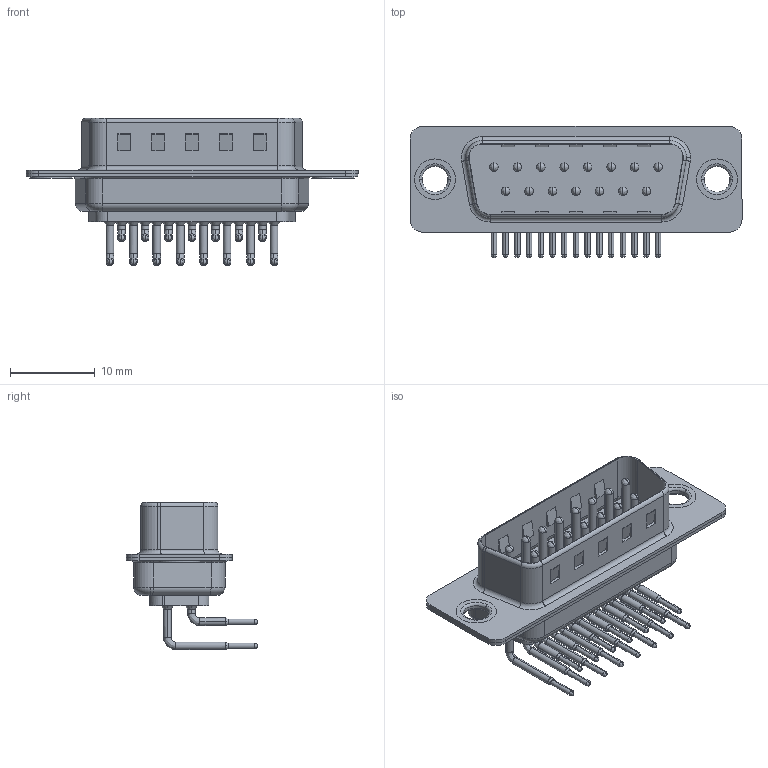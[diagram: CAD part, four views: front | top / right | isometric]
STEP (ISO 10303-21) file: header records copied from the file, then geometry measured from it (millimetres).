
FILE_DESCRIPTION (( 'STEP AP203' ), '1' );
FILE_NAME ('621-M15-360-BT1.STEP', '2018-09-24T23:09:31', ( '' ), ( '' ), 'SwSTEP 2.0', 'SolidWorks 2016', '' );
FILE_SCHEMA (( 'CONFIG_CONTROL_DESIGN' ));
Length unit declared in the file: millimetre
Products named in the file (7): 621M Thru Hole Rivet; 621-M15-360-BT1; 621M Housing_15 Contacts; 621M Shell Front_15 Contacts; 621M Shell Rear_15 Contacts; 621M Contact Row 1; 621M Contact Row 2
Assembly tree (20 placements, depth 2):
  621-M15-360-BT1
    621M Housing_15 Contacts
    621M Shell Front_15 Contacts
    621M Shell Rear_15 Contacts
    621M Contact Row 1  x8
    621M Contact Row 2  x7
    621M Thru Hole Rivet  x2
Bounding box: 39.2 x 15.49 x 17.39 mm (x, y, z)
Volume: 1858.8 mm3; surface area: 5111.4 mm2
Topology: 20 solids, 20 shells, 1964 faces, 5441 edges, 3528 vertices
Faces by surface type: plane 1099, cylinder 657, bspline 90, cone 60, torus 58
Entity records: 20277 total; most frequent: CARTESIAN_POINT 3488, DIRECTION 3441, ORIENTED_EDGE 3166, EDGE_CURVE 1583, AXIS2_PLACEMENT_3D 1244, VERTEX_POINT 1020, VECTOR 953, LINE 953
